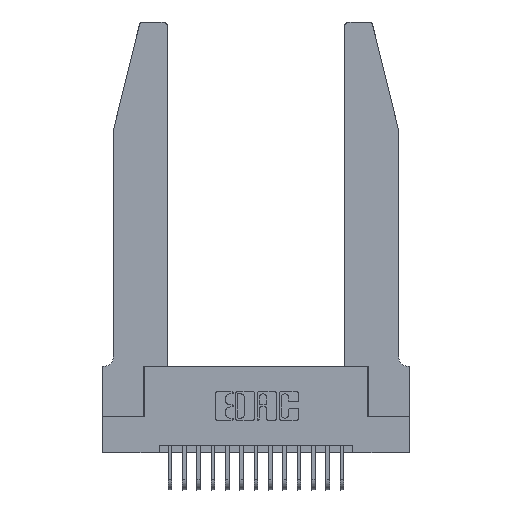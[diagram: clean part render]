
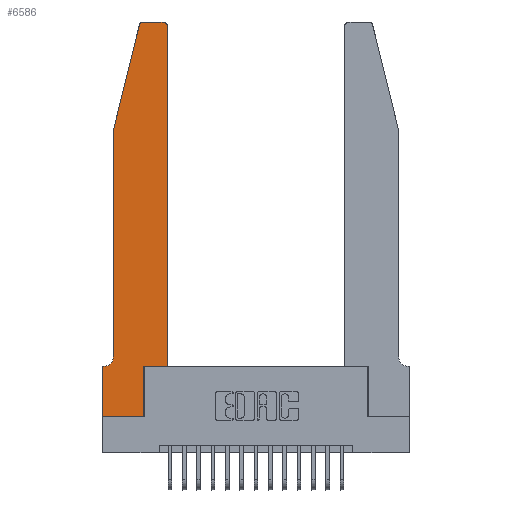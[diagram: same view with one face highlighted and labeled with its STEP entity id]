
A CAD part, top view. The second image highlights one B-rep face of the part: STEP entity #6586.
In plain terms, the highlighted planar face has unit normal (0, 0, 1).
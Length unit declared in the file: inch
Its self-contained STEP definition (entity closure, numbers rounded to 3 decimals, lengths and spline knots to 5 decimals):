
#3 = CARTESIAN_POINT ( 'NONE',  ( 0., 0., 0.37 ) ) ;
#227 = ORIENTED_EDGE ( 'NONE', *, *, #13657, .T. ) ;
#307 = VERTEX_POINT ( 'NONE', #10556 ) ;
#378 = ORIENTED_EDGE ( 'NONE', *, *, #623, .T. ) ;
#623 = EDGE_CURVE ( 'NONE', #10904, #1327, #4313, .T. ) ;
#885 = CARTESIAN_POINT ( 'NONE',  ( 0.0755, 0.42, 0.37 ) ) ;
#1249 = DIRECTION ( 'NONE',  ( 1., 0., 0. ) ) ;
#1257 = LINE ( 'NONE', #2514, #17596 ) ;
#1327 = VERTEX_POINT ( 'NONE', #8836 ) ;
#1784 = CARTESIAN_POINT ( 'NONE',  ( 0.284, 2.72, 0.37 ) ) ;
#1829 = CIRCLE ( 'NONE', #16037, 0.03 ) ;
#1967 = VERTEX_POINT ( 'NONE', #18443 ) ;
#2003 = CARTESIAN_POINT ( 'NONE',  ( 0.4205, 2.72, 0.37 ) ) ;
#2020 = CARTESIAN_POINT ( 'NONE',  ( 0.2605, 2.75, 0.37 ) ) ;
#2227 = CARTESIAN_POINT ( 'NONE',  ( 0.0755, 2., 0.37 ) ) ;
#2299 = ORIENTED_EDGE ( 'NONE', *, *, #9735, .T. ) ;
#2370 = LINE ( 'NONE', #17542, #19159 ) ;
#2389 = CARTESIAN_POINT ( 'NONE',  ( 0., 0., 0.37 ) ) ;
#2514 = CARTESIAN_POINT ( 'NONE',  ( 0.0755, 2., 0.37 ) ) ;
#2778 = PLANE ( 'NONE',  #18589 ) ;
#3274 = ORIENTED_EDGE ( 'NONE', *, *, #9281, .T. ) ;
#3365 = DIRECTION ( 'NONE',  ( 1., 0., 0. ) ) ;
#3477 = VERTEX_POINT ( 'NONE', #7827 ) ;
#3599 = DIRECTION ( 'NONE',  ( 1., 0., 0. ) ) ;
#3636 = CARTESIAN_POINT ( 'NONE',  ( 0.4505, 2.72, 0.37 ) ) ;
#3662 = VECTOR ( 'NONE', #19238, 39.37008 ) ;
#3710 = CARTESIAN_POINT ( 'NONE',  ( 0.4505, 0.35, 0.37 ) ) ;
#3808 = VECTOR ( 'NONE', #4107, 39.37008 ) ;
#3818 = DIRECTION ( 'NONE',  ( 0., -1., 0. ) ) ;
#3922 = VECTOR ( 'NONE', #8548, 39.37008 ) ;
#3944 = ORIENTED_EDGE ( 'NONE', *, *, #4520, .T. ) ;
#4107 = DIRECTION ( 'NONE',  ( 1., 0., 0. ) ) ;
#4313 = LINE ( 'NONE', #3, #3808 ) ;
#4366 = AXIS2_PLACEMENT_3D ( 'NONE', #17472, #7994, #19020 ) ;
#4520 = EDGE_CURVE ( 'NONE', #18772, #6398, #20030, .T. ) ;
#4655 = EDGE_CURVE ( 'NONE', #18542, #18772, #1257, .T. ) ;
#4901 = VECTOR ( 'NONE', #19849, 39.37008 ) ;
#5471 = ORIENTED_EDGE ( 'NONE', *, *, #6251, .T. ) ;
#6232 = ORIENTED_EDGE ( 'NONE', *, *, #14289, .T. ) ;
#6251 = EDGE_CURVE ( 'NONE', #15375, #18345, #12397, .T. ) ;
#6398 = VERTEX_POINT ( 'NONE', #885 ) ;
#6586 = ADVANCED_FACE ( 'NONE', ( #11146 ), #2778, .T. ) ;
#6609 = CARTESIAN_POINT ( 'NONE',  ( 0.2865, 0.35, 0.37 ) ) ;
#7827 = CARTESIAN_POINT ( 'NONE',  ( 0.284, 2.75, 0.37 ) ) ;
#7837 = VERTEX_POINT ( 'NONE', #18277 ) ;
#7994 = DIRECTION ( 'NONE',  ( 0., 0., -1. ) ) ;
#8071 = DIRECTION ( 'NONE',  ( 0., -1., 0. ) ) ;
#8123 = VERTEX_POINT ( 'NONE', #12996 ) ;
#8176 = EDGE_LOOP ( 'NONE', ( #15997, #17249, #13630, #3944, #16335, #6232, #3274, #378, #10990, #227, #5471, #2299 ) ) ;
#8548 = DIRECTION ( 'NONE',  ( 0., 1., 0. ) ) ;
#8836 = CARTESIAN_POINT ( 'NONE',  ( 0.2865, 0., 0.37 ) ) ;
#9281 = EDGE_CURVE ( 'NONE', #7837, #10904, #2370, .T. ) ;
#9427 = LINE ( 'NONE', #3710, #13150 ) ;
#9663 = CARTESIAN_POINT ( 'NONE',  ( 0.4505, 0.35, 0.37 ) ) ;
#9735 = EDGE_CURVE ( 'NONE', #18345, #307, #19142, .T. ) ;
#10130 = LINE ( 'NONE', #2020, #15328 ) ;
#10283 = EDGE_CURVE ( 'NONE', #3477, #18542, #1829, .T. ) ;
#10494 = DIRECTION ( 'NONE',  ( -0.239, -0.971, 0. ) ) ;
#10556 = CARTESIAN_POINT ( 'NONE',  ( 0.4205, 2.75, 0.37 ) ) ;
#10780 = DIRECTION ( 'NONE',  ( 0., 0., 1. ) ) ;
#10904 = VERTEX_POINT ( 'NONE', #2389 ) ;
#10990 = ORIENTED_EDGE ( 'NONE', *, *, #18320, .T. ) ;
#11013 = CARTESIAN_POINT ( 'NONE',  ( 0.0755, 2., 0.37 ) ) ;
#11146 = FACE_OUTER_BOUND ( 'NONE', #8176, .T. ) ;
#11551 = DIRECTION ( 'NONE',  ( -1., 0., 0. ) ) ;
#11641 = LINE ( 'NONE', #6609, #3662 ) ;
#11710 = VECTOR ( 'NONE', #3818, 39.37008 ) ;
#12066 = CARTESIAN_POINT ( 'NONE',  ( 0.25487, 2.72718, 0.37 ) ) ;
#12397 = LINE ( 'NONE', #14862, #3922 ) ;
#12791 = EDGE_CURVE ( 'NONE', #6398, #8123, #20489, .T. ) ;
#12896 = DIRECTION ( 'NONE',  ( 0., 0., 1. ) ) ;
#12996 = CARTESIAN_POINT ( 'NONE',  ( 0.0055, 0.35, 0.37 ) ) ;
#13125 = DIRECTION ( 'NONE',  ( 0., 0., 1. ) ) ;
#13150 = VECTOR ( 'NONE', #18030, 39.37008 ) ;
#13373 = LINE ( 'NONE', #16675, #4901 ) ;
#13630 = ORIENTED_EDGE ( 'NONE', *, *, #4655, .T. ) ;
#13657 = EDGE_CURVE ( 'NONE', #1967, #15375, #9427, .T. ) ;
#14289 = EDGE_CURVE ( 'NONE', #8123, #7837, #13373, .T. ) ;
#14700 = EDGE_CURVE ( 'NONE', #307, #3477, #10130, .T. ) ;
#14862 = CARTESIAN_POINT ( 'NONE',  ( 0.4505, 0.35, 0.37 ) ) ;
#15328 = VECTOR ( 'NONE', #11551, 39.37008 ) ;
#15375 = VERTEX_POINT ( 'NONE', #9663 ) ;
#15997 = ORIENTED_EDGE ( 'NONE', *, *, #14700, .T. ) ;
#16037 = AXIS2_PLACEMENT_3D ( 'NONE', #1784, #12896, #3365 ) ;
#16335 = ORIENTED_EDGE ( 'NONE', *, *, #12791, .T. ) ;
#16675 = CARTESIAN_POINT ( 'NONE',  ( 0.0755, 0.35, 0.37 ) ) ;
#16823 = AXIS2_PLACEMENT_3D ( 'NONE', #2003, #13125, #3599 ) ;
#17249 = ORIENTED_EDGE ( 'NONE', *, *, #10283, .T. ) ;
#17472 = CARTESIAN_POINT ( 'NONE',  ( 0.0055, 0.42, 0.37 ) ) ;
#17542 = CARTESIAN_POINT ( 'NONE',  ( 0., 0., 0.37 ) ) ;
#17596 = VECTOR ( 'NONE', #10494, 39.37008 ) ;
#18030 = DIRECTION ( 'NONE',  ( 1., 0., 0. ) ) ;
#18277 = CARTESIAN_POINT ( 'NONE',  ( 0., 0.35, 0.37 ) ) ;
#18320 = EDGE_CURVE ( 'NONE', #1327, #1967, #11641, .T. ) ;
#18345 = VERTEX_POINT ( 'NONE', #3636 ) ;
#18443 = CARTESIAN_POINT ( 'NONE',  ( 0.2865, 0.35, 0.37 ) ) ;
#18542 = VERTEX_POINT ( 'NONE', #12066 ) ;
#18589 = AXIS2_PLACEMENT_3D ( 'NONE', #20161, #10780, #1249 ) ;
#18772 = VERTEX_POINT ( 'NONE', #11013 ) ;
#19020 = DIRECTION ( 'NONE',  ( -1., 0., 0. ) ) ;
#19142 = CIRCLE ( 'NONE', #16823, 0.03 ) ;
#19159 = VECTOR ( 'NONE', #8071, 39.37008 ) ;
#19238 = DIRECTION ( 'NONE',  ( 0., 1., 0. ) ) ;
#19849 = DIRECTION ( 'NONE',  ( -1., 0., 0. ) ) ;
#20030 = LINE ( 'NONE', #2227, #11710 ) ;
#20161 = CARTESIAN_POINT ( 'NONE',  ( 0., 0.35, 0.37 ) ) ;
#20489 = CIRCLE ( 'NONE', #4366, 0.07 ) ;
